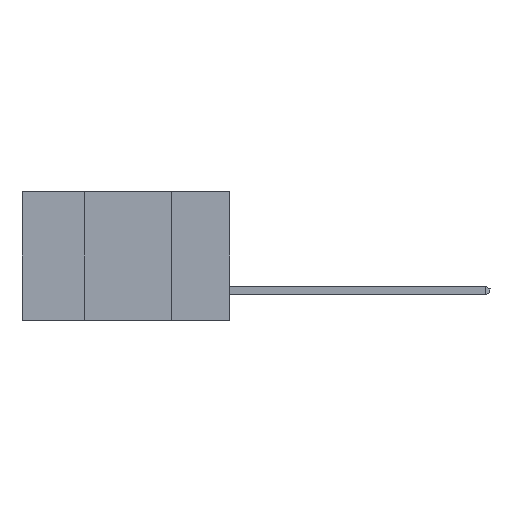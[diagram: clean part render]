
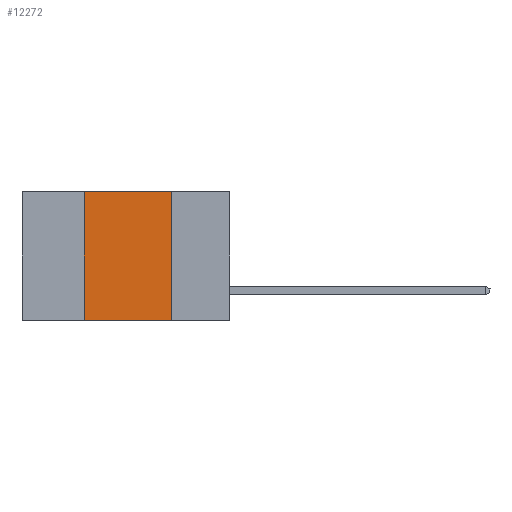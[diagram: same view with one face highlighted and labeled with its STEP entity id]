
A CAD part, left-side view. The second image highlights one B-rep face of the part: STEP entity #12272.
In plain terms, the highlighted planar face has unit normal (-1, 0, 0).
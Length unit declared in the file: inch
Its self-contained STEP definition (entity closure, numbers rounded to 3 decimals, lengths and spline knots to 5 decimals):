
#367 = LINE ( 'NONE', #4771, #6589 ) ;
#959 = AXIS2_PLACEMENT_3D ( 'NONE', #13204, #9972, #13270 ) ;
#1032 = CARTESIAN_POINT ( 'NONE',  ( 0., 0.17, -0.37 ) ) ;
#1725 = EDGE_CURVE ( 'NONE', #8528, #6169, #367, .T. ) ;
#1871 = ORIENTED_EDGE ( 'NONE', *, *, #4849, .F. ) ;
#1995 = VERTEX_POINT ( 'NONE', #4664 ) ;
#4277 = LINE ( 'NONE', #6379, #8785 ) ;
#4664 = CARTESIAN_POINT ( 'NONE',  ( 0., 0.42, 0. ) ) ;
#4771 = CARTESIAN_POINT ( 'NONE',  ( 0., 0.6, -0.37 ) ) ;
#4849 = EDGE_CURVE ( 'NONE', #6142, #6169, #4277, .T. ) ;
#6104 = DIRECTION ( 'NONE',  ( 0., 0., 1. ) ) ;
#6132 = EDGE_CURVE ( 'NONE', #8528, #1995, #12672, .T. ) ;
#6142 = VERTEX_POINT ( 'NONE', #11511 ) ;
#6169 = VERTEX_POINT ( 'NONE', #1032 ) ;
#6379 = CARTESIAN_POINT ( 'NONE',  ( 0., 0.17, -0.37 ) ) ;
#6589 = VECTOR ( 'NONE', #9176, 39.37008 ) ;
#6637 = PLANE ( 'NONE',  #959 ) ;
#7153 = ORIENTED_EDGE ( 'NONE', *, *, #1725, .T. ) ;
#8129 = EDGE_LOOP ( 'NONE', ( #1871, #13984, #9320, #7153 ) ) ;
#8208 = DIRECTION ( 'NONE',  ( 0., -1., 0. ) ) ;
#8528 = VERTEX_POINT ( 'NONE', #11121 ) ;
#8785 = VECTOR ( 'NONE', #12082, 39.37008 ) ;
#9109 = VECTOR ( 'NONE', #6104, 39.37008 ) ;
#9176 = DIRECTION ( 'NONE',  ( 0., -1., 0. ) ) ;
#9290 = CARTESIAN_POINT ( 'NONE',  ( 0., 0.6, 0. ) ) ;
#9320 = ORIENTED_EDGE ( 'NONE', *, *, #6132, .F. ) ;
#9640 = CARTESIAN_POINT ( 'NONE',  ( 0., 0.42, -0.37 ) ) ;
#9899 = FACE_OUTER_BOUND ( 'NONE', #8129, .T. ) ;
#9972 = DIRECTION ( 'NONE',  ( 1., 0., 0. ) ) ;
#10182 = VECTOR ( 'NONE', #8208, 39.37008 ) ;
#11121 = CARTESIAN_POINT ( 'NONE',  ( 0., 0.42, -0.37 ) ) ;
#11510 = EDGE_CURVE ( 'NONE', #1995, #6142, #12324, .T. ) ;
#11511 = CARTESIAN_POINT ( 'NONE',  ( 0., 0.17, 0. ) ) ;
#12082 = DIRECTION ( 'NONE',  ( 0., 0., -1. ) ) ;
#12272 = ADVANCED_FACE ( 'NONE', ( #9899 ), #6637, .F. ) ;
#12324 = LINE ( 'NONE', #9290, #10182 ) ;
#12672 = LINE ( 'NONE', #9640, #9109 ) ;
#13204 = CARTESIAN_POINT ( 'NONE',  ( 0., 0.6, 0. ) ) ;
#13270 = DIRECTION ( 'NONE',  ( 0., 0., -1. ) ) ;
#13984 = ORIENTED_EDGE ( 'NONE', *, *, #11510, .F. ) ;
